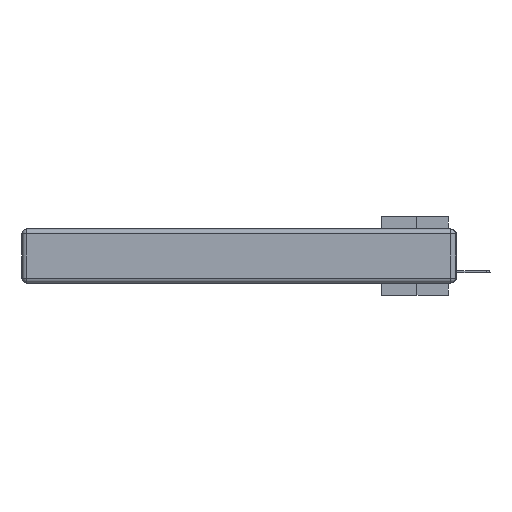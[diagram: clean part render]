
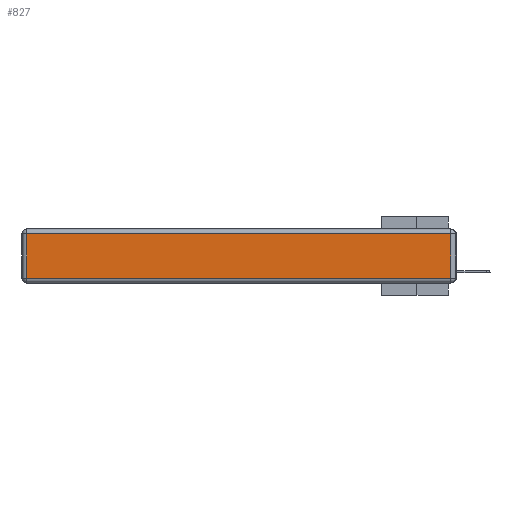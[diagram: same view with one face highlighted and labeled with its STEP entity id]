
A CAD part, left-side view. The second image highlights one B-rep face of the part: STEP entity #827.
In plain terms, the highlighted planar face has unit normal (-1, 0, 0).
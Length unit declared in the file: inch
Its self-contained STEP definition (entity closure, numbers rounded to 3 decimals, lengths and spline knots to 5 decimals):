
#827 = ADVANCED_FACE ( 'NONE', ( #23895 ), #15610, .T. ) ;
#2057 = VERTEX_POINT ( 'NONE', #8666 ) ;
#2599 = CARTESIAN_POINT ( 'NONE',  ( 0., 0., -0.313 ) ) ;
#2836 = CARTESIAN_POINT ( 'NONE',  ( 0., 0.03, -0.343 ) ) ;
#3808 = CARTESIAN_POINT ( 'NONE',  ( 0., 2.72, -0.343 ) ) ;
#3905 = AXIS2_PLACEMENT_3D ( 'NONE', #17854, #4476, #7458 ) ;
#4405 = LINE ( 'NONE', #11705, #13290 ) ;
#4476 = DIRECTION ( 'NONE',  ( -1., 0., 0. ) ) ;
#5433 = DIRECTION ( 'NONE',  ( 0., -1., 0. ) ) ;
#7303 = CARTESIAN_POINT ( 'NONE',  ( 0., 2.72, -0.313 ) ) ;
#7426 = EDGE_CURVE ( 'NONE', #2057, #16723, #22507, .T. ) ;
#7458 = DIRECTION ( 'NONE',  ( 0., 0., 1. ) ) ;
#8666 = CARTESIAN_POINT ( 'NONE',  ( 0., 2.72, -0.03 ) ) ;
#9101 = DIRECTION ( 'NONE',  ( 0., 1., 0. ) ) ;
#9420 = EDGE_CURVE ( 'NONE', #16723, #12186, #16888, .T. ) ;
#9846 = VERTEX_POINT ( 'NONE', #27965 ) ;
#11705 = CARTESIAN_POINT ( 'NONE',  ( 0., 2.75, -0.03 ) ) ;
#12186 = VERTEX_POINT ( 'NONE', #13955 ) ;
#12758 = ORIENTED_EDGE ( 'NONE', *, *, #9420, .T. ) ;
#13290 = VECTOR ( 'NONE', #9101, 39.37008 ) ;
#13955 = CARTESIAN_POINT ( 'NONE',  ( 0., 0.03, -0.313 ) ) ;
#15056 = VECTOR ( 'NONE', #29830, 39.37008 ) ;
#15610 = PLANE ( 'NONE',  #3905 ) ;
#16723 = VERTEX_POINT ( 'NONE', #7303 ) ;
#16888 = LINE ( 'NONE', #2599, #31790 ) ;
#17854 = CARTESIAN_POINT ( 'NONE',  ( 0., 0., -0.343 ) ) ;
#18582 = EDGE_CURVE ( 'NONE', #9846, #2057, #4405, .T. ) ;
#21657 = VECTOR ( 'NONE', #27567, 39.37008 ) ;
#22507 = LINE ( 'NONE', #3808, #21657 ) ;
#23261 = EDGE_LOOP ( 'NONE', ( #12758, #32450, #28902, #30249 ) ) ;
#23895 = FACE_OUTER_BOUND ( 'NONE', #23261, .T. ) ;
#27567 = DIRECTION ( 'NONE',  ( 0., 0., -1. ) ) ;
#27965 = CARTESIAN_POINT ( 'NONE',  ( 0., 0.03, -0.03 ) ) ;
#28902 = ORIENTED_EDGE ( 'NONE', *, *, #18582, .T. ) ;
#29814 = EDGE_CURVE ( 'NONE', #12186, #9846, #33726, .T. ) ;
#29830 = DIRECTION ( 'NONE',  ( 0., 0., 1. ) ) ;
#30249 = ORIENTED_EDGE ( 'NONE', *, *, #7426, .T. ) ;
#31790 = VECTOR ( 'NONE', #5433, 39.37008 ) ;
#32450 = ORIENTED_EDGE ( 'NONE', *, *, #29814, .T. ) ;
#33726 = LINE ( 'NONE', #2836, #15056 ) ;
